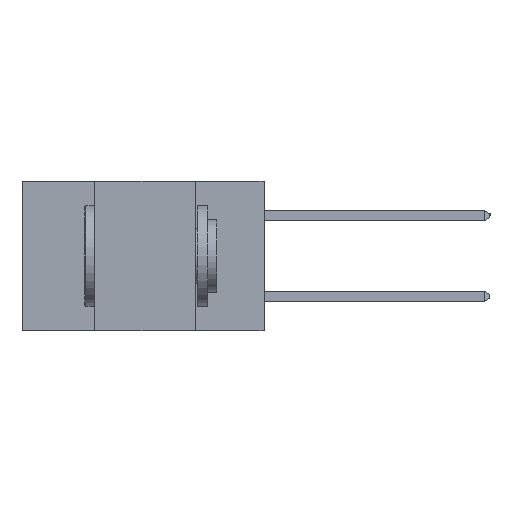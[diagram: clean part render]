
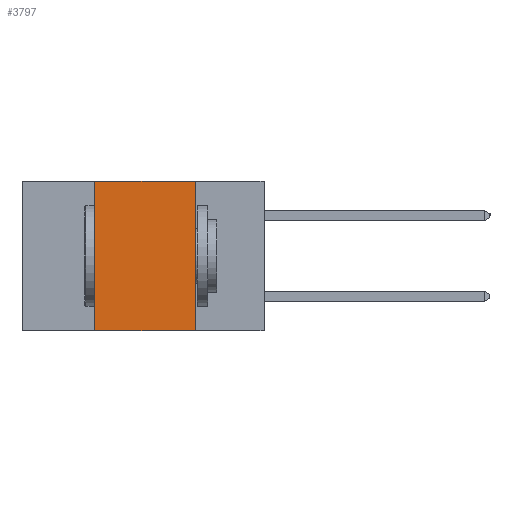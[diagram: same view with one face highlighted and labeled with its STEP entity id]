
A CAD part, left-side view. The second image highlights one B-rep face of the part: STEP entity #3797.
In plain terms, the highlighted planar face has unit normal (-1, 0, 0).
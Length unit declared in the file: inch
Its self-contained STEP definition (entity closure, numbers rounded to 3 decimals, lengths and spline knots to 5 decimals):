
#41 = ORIENTED_EDGE ( 'NONE', *, *, #9798, .F. ) ;
#1113 = VECTOR ( 'NONE', #5720, 39.37008 ) ;
#2040 = CARTESIAN_POINT ( 'NONE',  ( 0., 0.6, -0.37 ) ) ;
#2164 = VECTOR ( 'NONE', #11856, 39.37008 ) ;
#2170 = EDGE_LOOP ( 'NONE', ( #11539, #10451, #41, #12608 ) ) ;
#3494 = CARTESIAN_POINT ( 'NONE',  ( 0., 0.42, -0.37 ) ) ;
#3671 = DIRECTION ( 'NONE',  ( 0., 0., -1. ) ) ;
#3739 = FACE_OUTER_BOUND ( 'NONE', #2170, .T. ) ;
#3797 = ADVANCED_FACE ( 'NONE', ( #3739 ), #6957, .F. ) ;
#3799 = LINE ( 'NONE', #8926, #2164 ) ;
#3938 = CARTESIAN_POINT ( 'NONE',  ( 0., 0.6, 0. ) ) ;
#4274 = CARTESIAN_POINT ( 'NONE',  ( 0., 0.17, -0.37 ) ) ;
#5529 = LINE ( 'NONE', #3494, #1113 ) ;
#5720 = DIRECTION ( 'NONE',  ( 0., 0., 1. ) ) ;
#6106 = LINE ( 'NONE', #2040, #8034 ) ;
#6748 = CARTESIAN_POINT ( 'NONE',  ( 0., 0.42, 0. ) ) ;
#6759 = EDGE_CURVE ( 'NONE', #10539, #6913, #10826, .T. ) ;
#6841 = DIRECTION ( 'NONE',  ( 0., -1., 0. ) ) ;
#6913 = VERTEX_POINT ( 'NONE', #11994 ) ;
#6957 = PLANE ( 'NONE',  #11050 ) ;
#7359 = VECTOR ( 'NONE', #6841, 39.37008 ) ;
#7690 = DIRECTION ( 'NONE',  ( 1., 0., 0. ) ) ;
#7896 = CARTESIAN_POINT ( 'NONE',  ( 0., 0.42, -0.37 ) ) ;
#8034 = VECTOR ( 'NONE', #10050, 39.37008 ) ;
#8225 = VERTEX_POINT ( 'NONE', #4274 ) ;
#8926 = CARTESIAN_POINT ( 'NONE',  ( 0., 0.17, -0.37 ) ) ;
#9798 = EDGE_CURVE ( 'NONE', #11090, #10539, #5529, .T. ) ;
#10050 = DIRECTION ( 'NONE',  ( 0., -1., 0. ) ) ;
#10451 = ORIENTED_EDGE ( 'NONE', *, *, #6759, .F. ) ;
#10539 = VERTEX_POINT ( 'NONE', #6748 ) ;
#10826 = LINE ( 'NONE', #3938, #7359 ) ;
#11050 = AXIS2_PLACEMENT_3D ( 'NONE', #11793, #7690, #3671 ) ;
#11090 = VERTEX_POINT ( 'NONE', #7896 ) ;
#11291 = EDGE_CURVE ( 'NONE', #11090, #8225, #6106, .T. ) ;
#11539 = ORIENTED_EDGE ( 'NONE', *, *, #11576, .F. ) ;
#11576 = EDGE_CURVE ( 'NONE', #6913, #8225, #3799, .T. ) ;
#11793 = CARTESIAN_POINT ( 'NONE',  ( 0., 0.6, 0. ) ) ;
#11856 = DIRECTION ( 'NONE',  ( 0., 0., -1. ) ) ;
#11994 = CARTESIAN_POINT ( 'NONE',  ( 0., 0.17, 0. ) ) ;
#12608 = ORIENTED_EDGE ( 'NONE', *, *, #11291, .T. ) ;
